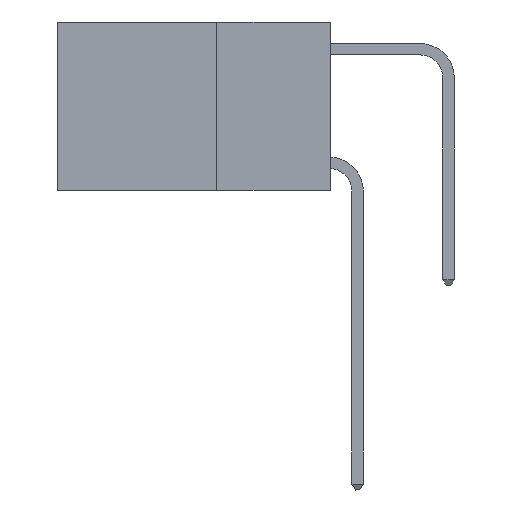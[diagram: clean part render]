
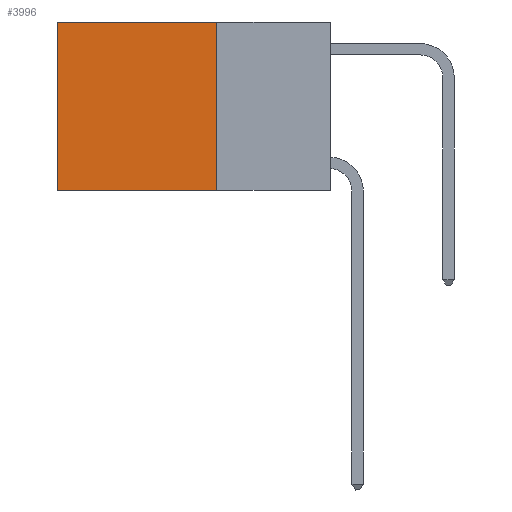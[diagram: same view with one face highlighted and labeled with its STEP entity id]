
A CAD part, left-side view. The second image highlights one B-rep face of the part: STEP entity #3996.
In plain terms, the highlighted planar face has unit normal (-1, 0, 0).
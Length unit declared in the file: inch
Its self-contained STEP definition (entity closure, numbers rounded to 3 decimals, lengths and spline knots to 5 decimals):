
#252 = EDGE_CURVE ( 'NONE', #11773, #9951, #1467, .T. ) ;
#355 = PLANE ( 'NONE',  #2788 ) ;
#1388 = DIRECTION ( 'NONE',  ( 0., 0., -1. ) ) ;
#1467 = LINE ( 'NONE', #5291, #9233 ) ;
#2003 = VECTOR ( 'NONE', #10868, 39.37008 ) ;
#2788 = AXIS2_PLACEMENT_3D ( 'NONE', #8431, #7468, #1388 ) ;
#2832 = EDGE_CURVE ( 'NONE', #11773, #7264, #12097, .T. ) ;
#3465 = VERTEX_POINT ( 'NONE', #11749 ) ;
#3996 = ADVANCED_FACE ( 'NONE', ( #7419 ), #355, .F. ) ;
#4536 = VECTOR ( 'NONE', #8803, 39.37008 ) ;
#4681 = CARTESIAN_POINT ( 'NONE',  ( 0.2625, 0.25, 0. ) ) ;
#4687 = CARTESIAN_POINT ( 'NONE',  ( 0.2625, 0.6, 0. ) ) ;
#5291 = CARTESIAN_POINT ( 'NONE',  ( 0.2625, 0.25, 0. ) ) ;
#5380 = ORIENTED_EDGE ( 'NONE', *, *, #7395, .T. ) ;
#5533 = ORIENTED_EDGE ( 'NONE', *, *, #6232, .F. ) ;
#5774 = ORIENTED_EDGE ( 'NONE', *, *, #252, .F. ) ;
#5925 = DIRECTION ( 'NONE',  ( 0., 0., -1. ) ) ;
#6138 = ORIENTED_EDGE ( 'NONE', *, *, #2832, .T. ) ;
#6232 = EDGE_CURVE ( 'NONE', #9951, #3465, #7292, .T. ) ;
#6974 = VECTOR ( 'NONE', #9914, 39.37008 ) ;
#7264 = VERTEX_POINT ( 'NONE', #12659 ) ;
#7292 = LINE ( 'NONE', #12848, #4536 ) ;
#7395 = EDGE_CURVE ( 'NONE', #7264, #3465, #13114, .T. ) ;
#7419 = FACE_OUTER_BOUND ( 'NONE', #10046, .T. ) ;
#7468 = DIRECTION ( 'NONE',  ( 1., 0., 0. ) ) ;
#8431 = CARTESIAN_POINT ( 'NONE',  ( 0.2625, 0.25, 0. ) ) ;
#8803 = DIRECTION ( 'NONE',  ( 0., 1., 0. ) ) ;
#9233 = VECTOR ( 'NONE', #5925, 39.37008 ) ;
#9914 = DIRECTION ( 'NONE',  ( 0., 1., 0. ) ) ;
#9951 = VERTEX_POINT ( 'NONE', #12856 ) ;
#10040 = CARTESIAN_POINT ( 'NONE',  ( 0.2625, 0.25, 0. ) ) ;
#10046 = EDGE_LOOP ( 'NONE', ( #5380, #5533, #5774, #6138 ) ) ;
#10868 = DIRECTION ( 'NONE',  ( 0., 0., -1. ) ) ;
#11749 = CARTESIAN_POINT ( 'NONE',  ( 0.2625, 0.6, -0.37 ) ) ;
#11773 = VERTEX_POINT ( 'NONE', #4681 ) ;
#12097 = LINE ( 'NONE', #10040, #6974 ) ;
#12659 = CARTESIAN_POINT ( 'NONE',  ( 0.2625, 0.6, 0. ) ) ;
#12848 = CARTESIAN_POINT ( 'NONE',  ( 0.2625, 0.25, -0.37 ) ) ;
#12856 = CARTESIAN_POINT ( 'NONE',  ( 0.2625, 0.25, -0.37 ) ) ;
#13114 = LINE ( 'NONE', #4687, #2003 ) ;
